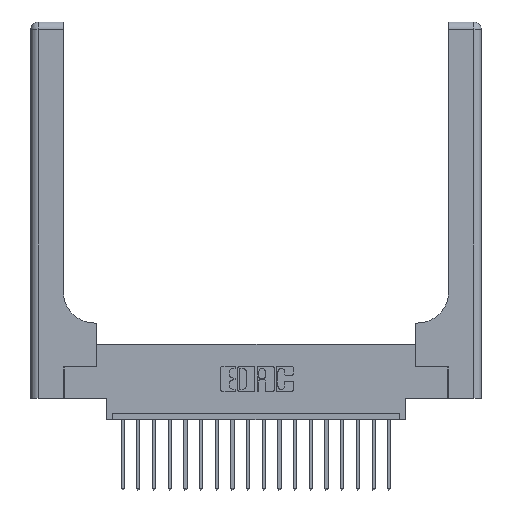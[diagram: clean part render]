
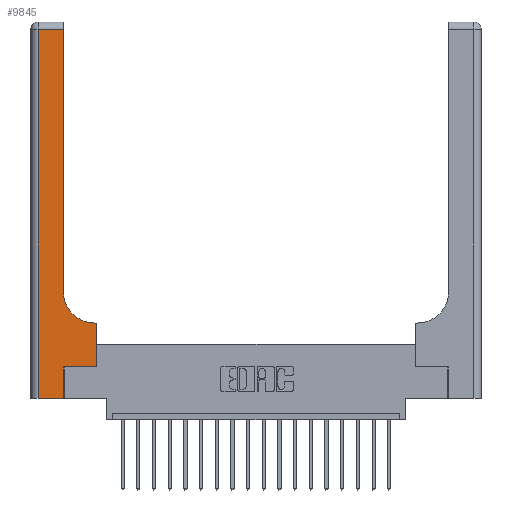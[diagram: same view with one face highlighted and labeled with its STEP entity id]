
A CAD part, top view. The second image highlights one B-rep face of the part: STEP entity #9845.
In plain terms, the highlighted planar face has unit normal (0, 0, 1).
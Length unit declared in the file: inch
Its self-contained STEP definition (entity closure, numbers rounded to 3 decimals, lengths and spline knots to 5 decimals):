
#20 = CARTESIAN_POINT ( 'NONE',  ( 0.26, 0.6, 0.37 ) ) ;
#322 = LINE ( 'NONE', #20, #10502 ) ;
#1062 = CARTESIAN_POINT ( 'NONE',  ( 0.51, 0.6, 0.37 ) ) ;
#1261 = PLANE ( 'NONE',  #6201 ) ;
#1455 = CARTESIAN_POINT ( 'NONE',  ( 0.528, 0.25, 0.37 ) ) ;
#2142 = CARTESIAN_POINT ( 'NONE',  ( 0.06, 0., 0.37 ) ) ;
#2378 = VECTOR ( 'NONE', #17101, 39.37008 ) ;
#2501 = DIRECTION ( 'NONE',  ( 0., 1., 0. ) ) ;
#2856 = DIRECTION ( 'NONE',  ( 0., 1., 0. ) ) ;
#2978 = DIRECTION ( 'NONE',  ( -1., 0., 0. ) ) ;
#3511 = VERTEX_POINT ( 'NONE', #2142 ) ;
#3651 = CARTESIAN_POINT ( 'NONE',  ( 0.265, 0., 0.37 ) ) ;
#3737 = ORIENTED_EDGE ( 'NONE', *, *, #8848, .T. ) ;
#3963 = ORIENTED_EDGE ( 'NONE', *, *, #5656, .T. ) ;
#4084 = LINE ( 'NONE', #19708, #8792 ) ;
#4222 = CARTESIAN_POINT ( 'NONE',  ( 0.265, 0., 0.37 ) ) ;
#4229 = VERTEX_POINT ( 'NONE', #7302 ) ;
#4335 = VECTOR ( 'NONE', #15592, 39.37008 ) ;
#5139 = VERTEX_POINT ( 'NONE', #19095 ) ;
#5312 = DIRECTION ( 'NONE',  ( 0., -1., 0. ) ) ;
#5466 = LINE ( 'NONE', #4222, #16858 ) ;
#5626 = CARTESIAN_POINT ( 'NONE',  ( 0.528, 0.25, 0.37 ) ) ;
#5644 = FACE_OUTER_BOUND ( 'NONE', #6396, .T. ) ;
#5656 = EDGE_CURVE ( 'NONE', #10447, #20121, #5466, .T. ) ;
#5749 = DIRECTION ( 'NONE',  ( 0., 0., -1. ) ) ;
#5818 = DIRECTION ( 'NONE',  ( 1., 0., 0. ) ) ;
#6013 = ORIENTED_EDGE ( 'NONE', *, *, #8874, .T. ) ;
#6071 = LINE ( 'NONE', #9226, #2378 ) ;
#6201 = AXIS2_PLACEMENT_3D ( 'NONE', #12269, #5749, #2978 ) ;
#6396 = EDGE_LOOP ( 'NONE', ( #6013, #18011, #3737, #10179, #3963, #19794, #6450, #20065, #11239 ) ) ;
#6450 = ORIENTED_EDGE ( 'NONE', *, *, #7429, .T. ) ;
#6698 = EDGE_CURVE ( 'NONE', #3511, #10447, #12435, .T. ) ;
#7302 = CARTESIAN_POINT ( 'NONE',  ( 0.26, 2.94, 0.37 ) ) ;
#7429 = EDGE_CURVE ( 'NONE', #18484, #5139, #20025, .T. ) ;
#7657 = DIRECTION ( 'NONE',  ( 0., 0., -1. ) ) ;
#7951 = CARTESIAN_POINT ( 'NONE',  ( 0.51, 0.85, 0.37 ) ) ;
#8660 = CARTESIAN_POINT ( 'NONE',  ( 0.26, 0.85, 0.37 ) ) ;
#8792 = VECTOR ( 'NONE', #2856, 39.37008 ) ;
#8848 = EDGE_CURVE ( 'NONE', #11008, #3511, #17483, .T. ) ;
#8874 = EDGE_CURVE ( 'NONE', #11364, #4229, #4084, .T. ) ;
#9169 = CIRCLE ( 'NONE', #14716, 0.25 ) ;
#9226 = CARTESIAN_POINT ( 'NONE',  ( 0.265, 0.25, 0.37 ) ) ;
#9845 = ADVANCED_FACE ( 'NONE', ( #5644 ), #1261, .F. ) ;
#10179 = ORIENTED_EDGE ( 'NONE', *, *, #6698, .T. ) ;
#10447 = VERTEX_POINT ( 'NONE', #3651 ) ;
#10502 = VECTOR ( 'NONE', #15747, 39.37008 ) ;
#10662 = CARTESIAN_POINT ( 'NONE',  ( 0.06, 2.94, 0.37 ) ) ;
#11008 = VERTEX_POINT ( 'NONE', #10662 ) ;
#11239 = ORIENTED_EDGE ( 'NONE', *, *, #12681, .T. ) ;
#11364 = VERTEX_POINT ( 'NONE', #8660 ) ;
#12269 = CARTESIAN_POINT ( 'NONE',  ( 0., 3., 0.37 ) ) ;
#12353 = DIRECTION ( 'NONE',  ( 1., 0., 0. ) ) ;
#12435 = LINE ( 'NONE', #13770, #14581 ) ;
#12681 = EDGE_CURVE ( 'NONE', #16834, #11364, #9169, .T. ) ;
#12887 = CARTESIAN_POINT ( 'NONE',  ( 0., 2.94, 0.37 ) ) ;
#13770 = CARTESIAN_POINT ( 'NONE',  ( 0., 0., 0.37 ) ) ;
#13902 = DIRECTION ( 'NONE',  ( 0., 1., 0. ) ) ;
#13958 = EDGE_CURVE ( 'NONE', #5139, #16834, #322, .T. ) ;
#14581 = VECTOR ( 'NONE', #5818, 39.37008 ) ;
#14716 = AXIS2_PLACEMENT_3D ( 'NONE', #7951, #7657, #12353 ) ;
#14840 = EDGE_CURVE ( 'NONE', #4229, #11008, #19020, .T. ) ;
#15232 = EDGE_CURVE ( 'NONE', #20121, #18484, #6071, .T. ) ;
#15449 = CARTESIAN_POINT ( 'NONE',  ( 0.265, 0.25, 0.37 ) ) ;
#15592 = DIRECTION ( 'NONE',  ( -1., 0., 0. ) ) ;
#15747 = DIRECTION ( 'NONE',  ( -1., 0., 0. ) ) ;
#15947 = CARTESIAN_POINT ( 'NONE',  ( 0.06, 3., 0.37 ) ) ;
#16834 = VERTEX_POINT ( 'NONE', #1062 ) ;
#16858 = VECTOR ( 'NONE', #2501, 39.37008 ) ;
#17101 = DIRECTION ( 'NONE',  ( 1., 0., 0. ) ) ;
#17483 = LINE ( 'NONE', #15947, #19562 ) ;
#18011 = ORIENTED_EDGE ( 'NONE', *, *, #14840, .T. ) ;
#18484 = VERTEX_POINT ( 'NONE', #5626 ) ;
#18544 = VECTOR ( 'NONE', #13902, 39.37008 ) ;
#19020 = LINE ( 'NONE', #12887, #4335 ) ;
#19095 = CARTESIAN_POINT ( 'NONE',  ( 0.528, 0.6, 0.37 ) ) ;
#19562 = VECTOR ( 'NONE', #5312, 39.37008 ) ;
#19708 = CARTESIAN_POINT ( 'NONE',  ( 0.26, 3., 0.37 ) ) ;
#19794 = ORIENTED_EDGE ( 'NONE', *, *, #15232, .T. ) ;
#20025 = LINE ( 'NONE', #1455, #18544 ) ;
#20065 = ORIENTED_EDGE ( 'NONE', *, *, #13958, .T. ) ;
#20121 = VERTEX_POINT ( 'NONE', #15449 ) ;
